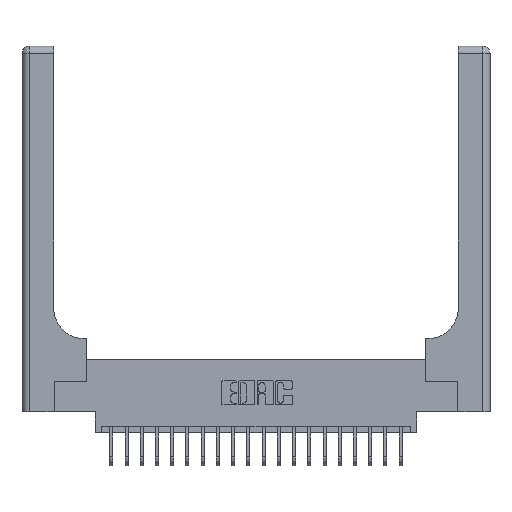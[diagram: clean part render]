
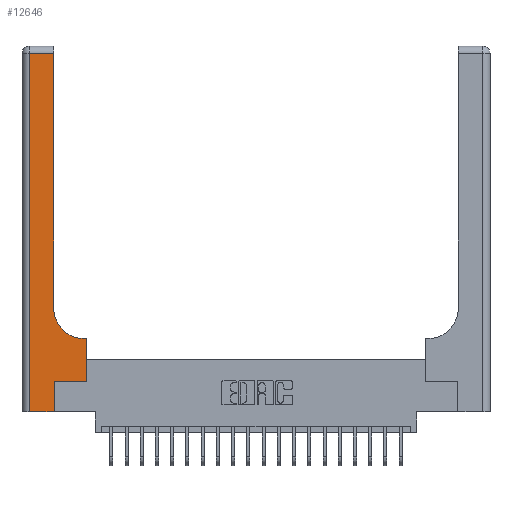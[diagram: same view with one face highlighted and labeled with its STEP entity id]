
A CAD part, top view. The second image highlights one B-rep face of the part: STEP entity #12646.
In plain terms, the highlighted planar face has unit normal (0, 0, 1).
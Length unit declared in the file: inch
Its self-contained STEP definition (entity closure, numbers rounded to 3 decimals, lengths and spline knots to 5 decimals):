
#111 = CARTESIAN_POINT ( 'NONE',  ( 0.265, 0., 0.37 ) ) ;
#534 = EDGE_CURVE ( 'NONE', #9383, #7241, #2008, .T. ) ;
#885 = CARTESIAN_POINT ( 'NONE',  ( 0.06, 2.94, 0.37 ) ) ;
#1981 = DIRECTION ( 'NONE',  ( -1., 0., 0. ) ) ;
#2008 = LINE ( 'NONE', #3674, #23184 ) ;
#2144 = VECTOR ( 'NONE', #14415, 39.37008 ) ;
#2993 = DIRECTION ( 'NONE',  ( 0., 1., 0. ) ) ;
#3443 = EDGE_CURVE ( 'NONE', #9322, #3462, #12715, .T. ) ;
#3462 = VERTEX_POINT ( 'NONE', #9146 ) ;
#3674 = CARTESIAN_POINT ( 'NONE',  ( 0.26, 0.6, 0.37 ) ) ;
#3779 = FACE_OUTER_BOUND ( 'NONE', #13349, .T. ) ;
#3803 = DIRECTION ( 'NONE',  ( -1., 0., 0. ) ) ;
#3926 = LINE ( 'NONE', #111, #14016 ) ;
#4003 = CARTESIAN_POINT ( 'NONE',  ( 0., 0., 0.37 ) ) ;
#4056 = CARTESIAN_POINT ( 'NONE',  ( 0.26, 0.85, 0.37 ) ) ;
#4143 = CARTESIAN_POINT ( 'NONE',  ( 0.265, 0.25, 0.37 ) ) ;
#4260 = CIRCLE ( 'NONE', #17582, 0.25 ) ;
#4323 = VERTEX_POINT ( 'NONE', #4056 ) ;
#4590 = ORIENTED_EDGE ( 'NONE', *, *, #10011, .T. ) ;
#5456 = CARTESIAN_POINT ( 'NONE',  ( 0.26, 3., 0.37 ) ) ;
#5475 = DIRECTION ( 'NONE',  ( 0., 1., 0. ) ) ;
#5905 = DIRECTION ( 'NONE',  ( 1., 0., 0. ) ) ;
#6178 = ORIENTED_EDGE ( 'NONE', *, *, #16775, .T. ) ;
#6320 = CARTESIAN_POINT ( 'NONE',  ( 0.528, 0.25, 0.37 ) ) ;
#6383 = EDGE_CURVE ( 'NONE', #7241, #4323, #4260, .T. ) ;
#6458 = VERTEX_POINT ( 'NONE', #17000 ) ;
#6843 = DIRECTION ( 'NONE',  ( 1., 0., 0. ) ) ;
#6956 = LINE ( 'NONE', #15676, #20835 ) ;
#7114 = LINE ( 'NONE', #5456, #2144 ) ;
#7238 = ORIENTED_EDGE ( 'NONE', *, *, #13340, .T. ) ;
#7241 = VERTEX_POINT ( 'NONE', #8715 ) ;
#7264 = CARTESIAN_POINT ( 'NONE',  ( 0.06, 0., 0.37 ) ) ;
#7956 = ORIENTED_EDGE ( 'NONE', *, *, #6383, .T. ) ;
#8242 = VECTOR ( 'NONE', #10083, 39.37008 ) ;
#8320 = EDGE_CURVE ( 'NONE', #9165, #11281, #13343, .T. ) ;
#8715 = CARTESIAN_POINT ( 'NONE',  ( 0.51, 0.6, 0.37 ) ) ;
#9033 = EDGE_CURVE ( 'NONE', #11281, #9322, #20320, .T. ) ;
#9146 = CARTESIAN_POINT ( 'NONE',  ( 0.265, 0., 0.37 ) ) ;
#9165 = VERTEX_POINT ( 'NONE', #12514 ) ;
#9295 = EDGE_CURVE ( 'NONE', #3462, #22744, #3926, .T. ) ;
#9322 = VERTEX_POINT ( 'NONE', #7264 ) ;
#9383 = VERTEX_POINT ( 'NONE', #22292 ) ;
#10011 = EDGE_CURVE ( 'NONE', #22744, #6458, #6956, .T. ) ;
#10083 = DIRECTION ( 'NONE',  ( -1., 0., 0. ) ) ;
#10198 = ORIENTED_EDGE ( 'NONE', *, *, #9295, .T. ) ;
#11153 = PLANE ( 'NONE',  #12386 ) ;
#11281 = VERTEX_POINT ( 'NONE', #885 ) ;
#11639 = VECTOR ( 'NONE', #2993, 39.37008 ) ;
#12266 = ORIENTED_EDGE ( 'NONE', *, *, #534, .T. ) ;
#12386 = AXIS2_PLACEMENT_3D ( 'NONE', #12590, #18435, #1981 ) ;
#12514 = CARTESIAN_POINT ( 'NONE',  ( 0.26, 2.94, 0.37 ) ) ;
#12587 = ORIENTED_EDGE ( 'NONE', *, *, #8320, .T. ) ;
#12590 = CARTESIAN_POINT ( 'NONE',  ( 0., 3., 0.37 ) ) ;
#12646 = ADVANCED_FACE ( 'NONE', ( #3779 ), #11153, .F. ) ;
#12715 = LINE ( 'NONE', #4003, #22115 ) ;
#13340 = EDGE_CURVE ( 'NONE', #6458, #9383, #15756, .T. ) ;
#13343 = LINE ( 'NONE', #20951, #8242 ) ;
#13349 = EDGE_LOOP ( 'NONE', ( #6178, #12587, #14334, #21452, #10198, #4590, #7238, #12266, #7956 ) ) ;
#13593 = CARTESIAN_POINT ( 'NONE',  ( 0.06, 3., 0.37 ) ) ;
#14016 = VECTOR ( 'NONE', #5475, 39.37008 ) ;
#14334 = ORIENTED_EDGE ( 'NONE', *, *, #9033, .T. ) ;
#14415 = DIRECTION ( 'NONE',  ( 0., 1., 0. ) ) ;
#14991 = DIRECTION ( 'NONE',  ( 1., 0., 0. ) ) ;
#15324 = DIRECTION ( 'NONE',  ( 0., 0., -1. ) ) ;
#15676 = CARTESIAN_POINT ( 'NONE',  ( 0.265, 0.25, 0.37 ) ) ;
#15756 = LINE ( 'NONE', #6320, #11639 ) ;
#16737 = VECTOR ( 'NONE', #19303, 39.37008 ) ;
#16775 = EDGE_CURVE ( 'NONE', #4323, #9165, #7114, .T. ) ;
#17000 = CARTESIAN_POINT ( 'NONE',  ( 0.528, 0.25, 0.37 ) ) ;
#17582 = AXIS2_PLACEMENT_3D ( 'NONE', #22256, #15324, #5905 ) ;
#18435 = DIRECTION ( 'NONE',  ( 0., 0., -1. ) ) ;
#19303 = DIRECTION ( 'NONE',  ( 0., -1., 0. ) ) ;
#20320 = LINE ( 'NONE', #13593, #16737 ) ;
#20835 = VECTOR ( 'NONE', #6843, 39.37008 ) ;
#20951 = CARTESIAN_POINT ( 'NONE',  ( 0., 2.94, 0.37 ) ) ;
#21452 = ORIENTED_EDGE ( 'NONE', *, *, #3443, .T. ) ;
#22115 = VECTOR ( 'NONE', #14991, 39.37008 ) ;
#22256 = CARTESIAN_POINT ( 'NONE',  ( 0.51, 0.85, 0.37 ) ) ;
#22292 = CARTESIAN_POINT ( 'NONE',  ( 0.528, 0.6, 0.37 ) ) ;
#22744 = VERTEX_POINT ( 'NONE', #4143 ) ;
#23184 = VECTOR ( 'NONE', #3803, 39.37008 ) ;
